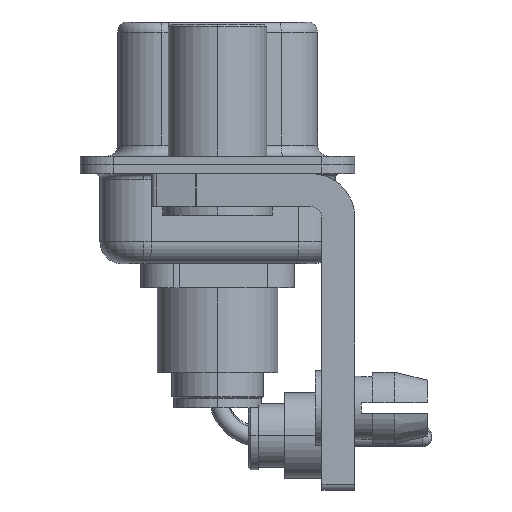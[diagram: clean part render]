
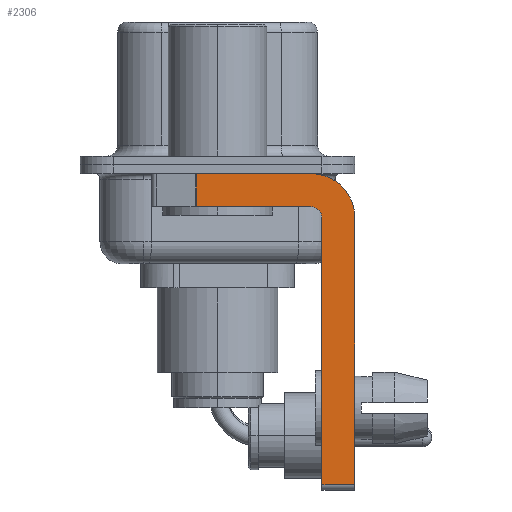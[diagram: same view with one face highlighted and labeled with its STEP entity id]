
A CAD part, left-side view. The second image highlights one B-rep face of the part: STEP entity #2306.
In plain terms, the highlighted planar face has unit normal (-1, 0, 0).
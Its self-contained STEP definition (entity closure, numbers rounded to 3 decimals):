
#53 = DIRECTION ( 'NONE',  ( 0., 1., 0. ) ) ;
#94 = EDGE_CURVE ( 'NONE', #9067, #21124, #5136, .T. ) ;
#557 = DIRECTION ( 'NONE',  ( 0., 0., 1. ) ) ;
#769 = VERTEX_POINT ( 'NONE', #1371 ) ;
#983 = ORIENTED_EDGE ( 'NONE', *, *, #19584, .F. ) ;
#985 = CARTESIAN_POINT ( 'NONE',  ( -2.9, 0.978, -0.4 ) ) ;
#1362 = EDGE_CURVE ( 'NONE', #3784, #17049, #17081, .T. ) ;
#1371 = CARTESIAN_POINT ( 'NONE',  ( -2.9, -6.25, -14.55 ) ) ;
#1808 = EDGE_CURVE ( 'NONE', #17049, #15860, #18669, .T. ) ;
#2238 = CARTESIAN_POINT ( 'NONE',  ( -2.9, -6.25, -2.4 ) ) ;
#2306 = ADVANCED_FACE ( 'NONE', ( #21095 ), #7160, .F. ) ;
#2356 = EDGE_LOOP ( 'NONE', ( #2382, #2815, #15679, #5912, #983, #12573, #20981, #6656 ) ) ;
#2382 = ORIENTED_EDGE ( 'NONE', *, *, #7843, .F. ) ;
#2815 = ORIENTED_EDGE ( 'NONE', *, *, #5927, .T. ) ;
#2950 = AXIS2_PLACEMENT_3D ( 'NONE', #9235, #5838, #19765 ) ;
#3237 = VECTOR ( 'NONE', #19483, 1000. ) ;
#3255 = CARTESIAN_POINT ( 'NONE',  ( -2.9, -4.25, -0.4 ) ) ;
#3286 = DIRECTION ( 'NONE',  ( -1., 0., 0. ) ) ;
#3412 = CARTESIAN_POINT ( 'NONE',  ( -2.9, -4.25, -2.4 ) ) ;
#3434 = VECTOR ( 'NONE', #557, 1000. ) ;
#3522 = DIRECTION ( 'NONE',  ( 1., 0., 0. ) ) ;
#3728 = CARTESIAN_POINT ( 'NONE',  ( -2.9, 0.978, -1.9 ) ) ;
#3784 = VERTEX_POINT ( 'NONE', #17060 ) ;
#4428 = LINE ( 'NONE', #21867, #12132 ) ;
#5136 = CIRCLE ( 'NONE', #2950, 2. ) ;
#5300 = CARTESIAN_POINT ( 'NONE',  ( -2.9, -4.25, -2.4 ) ) ;
#5317 = VECTOR ( 'NONE', #20971, 1000. ) ;
#5838 = DIRECTION ( 'NONE',  ( 1., 0., 0. ) ) ;
#5912 = ORIENTED_EDGE ( 'NONE', *, *, #1362, .F. ) ;
#5927 = EDGE_CURVE ( 'NONE', #7572, #15860, #10973, .T. ) ;
#6656 = ORIENTED_EDGE ( 'NONE', *, *, #94, .F. ) ;
#6743 = CARTESIAN_POINT ( 'NONE',  ( -2.9, -4.25, -1.9 ) ) ;
#7160 = PLANE ( 'NONE',  #16346 ) ;
#7316 = AXIS2_PLACEMENT_3D ( 'NONE', #5300, #3286, #22293 ) ;
#7572 = VERTEX_POINT ( 'NONE', #985 ) ;
#7843 = EDGE_CURVE ( 'NONE', #7572, #9067, #20952, .T. ) ;
#9067 = VERTEX_POINT ( 'NONE', #3255 ) ;
#9235 = CARTESIAN_POINT ( 'NONE',  ( -2.9, -4.25, -2.4 ) ) ;
#9253 = CARTESIAN_POINT ( 'NONE',  ( -2.9, 3., -0.4 ) ) ;
#10446 = DIRECTION ( 'NONE',  ( 0., 0., -1. ) ) ;
#10928 = CARTESIAN_POINT ( 'NONE',  ( -2.9, -6.25, -2.4 ) ) ;
#10973 = LINE ( 'NONE', #3728, #5317 ) ;
#11233 = DIRECTION ( 'NONE',  ( 0., -1., 0. ) ) ;
#11267 = VECTOR ( 'NONE', #53, 1000. ) ;
#12132 = VECTOR ( 'NONE', #11233, 1000. ) ;
#12573 = ORIENTED_EDGE ( 'NONE', *, *, #19775, .T. ) ;
#15679 = ORIENTED_EDGE ( 'NONE', *, *, #1808, .F. ) ;
#15860 = VERTEX_POINT ( 'NONE', #18906 ) ;
#16211 = LINE ( 'NONE', #19399, #3434 ) ;
#16346 = AXIS2_PLACEMENT_3D ( 'NONE', #3412, #3522, #10446 ) ;
#16968 = CARTESIAN_POINT ( 'NONE',  ( -2.9, -4.25, -1.9 ) ) ;
#17049 = VERTEX_POINT ( 'NONE', #6743 ) ;
#17060 = CARTESIAN_POINT ( 'NONE',  ( -2.9, -4.75, -2.4 ) ) ;
#17081 = CIRCLE ( 'NONE', #7316, 0.5 ) ;
#17660 = LINE ( 'NONE', #2238, #3237 ) ;
#18669 = LINE ( 'NONE', #16968, #11267 ) ;
#18735 = EDGE_CURVE ( 'NONE', #21124, #769, #17660, .T. ) ;
#18906 = CARTESIAN_POINT ( 'NONE',  ( -2.9, 0.978, -1.9 ) ) ;
#18995 = CARTESIAN_POINT ( 'NONE',  ( -2.9, -4.75, -14.55 ) ) ;
#18999 = VERTEX_POINT ( 'NONE', #18995 ) ;
#19399 = CARTESIAN_POINT ( 'NONE',  ( -2.9, -4.75, -14.8 ) ) ;
#19483 = DIRECTION ( 'NONE',  ( 0., 0., -1. ) ) ;
#19584 = EDGE_CURVE ( 'NONE', #18999, #3784, #16211, .T. ) ;
#19765 = DIRECTION ( 'NONE',  ( 0., 0., -1. ) ) ;
#19775 = EDGE_CURVE ( 'NONE', #18999, #769, #4428, .T. ) ;
#20952 = LINE ( 'NONE', #9253, #21323 ) ;
#20971 = DIRECTION ( 'NONE',  ( 0., 0., -1. ) ) ;
#20981 = ORIENTED_EDGE ( 'NONE', *, *, #18735, .F. ) ;
#21095 = FACE_OUTER_BOUND ( 'NONE', #2356, .T. ) ;
#21124 = VERTEX_POINT ( 'NONE', #10928 ) ;
#21159 = DIRECTION ( 'NONE',  ( 0., -1., 0. ) ) ;
#21323 = VECTOR ( 'NONE', #21159, 1000. ) ;
#21867 = CARTESIAN_POINT ( 'NONE',  ( -2.9, -4.25, -14.55 ) ) ;
#22293 = DIRECTION ( 'NONE',  ( 0., 0., 1. ) ) ;
